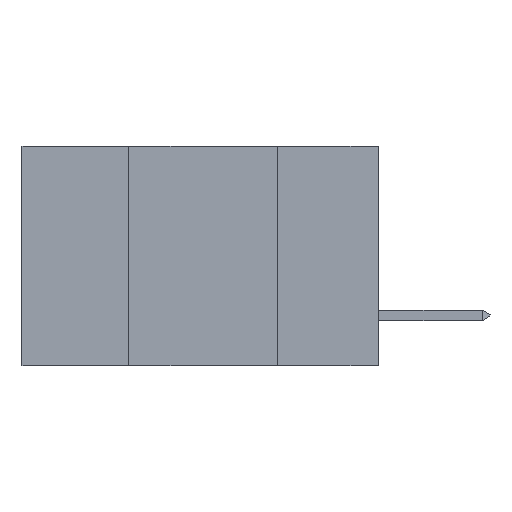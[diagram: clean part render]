
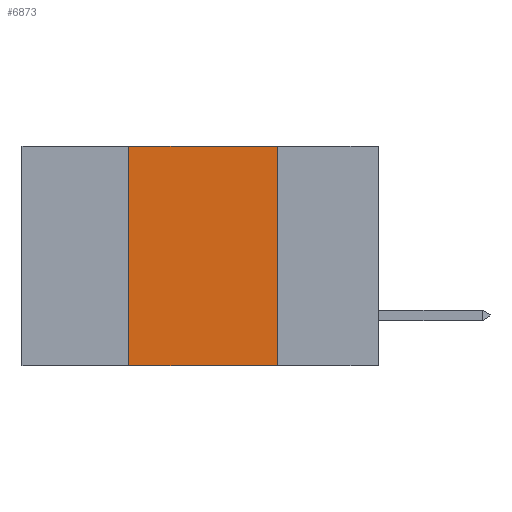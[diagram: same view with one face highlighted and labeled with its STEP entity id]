
A CAD part, left-side view. The second image highlights one B-rep face of the part: STEP entity #6873.
In plain terms, the highlighted planar face has unit normal (-1, 0, 0).
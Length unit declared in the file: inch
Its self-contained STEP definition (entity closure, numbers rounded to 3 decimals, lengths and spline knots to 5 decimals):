
#1115 = DIRECTION ( 'NONE',  ( 0., -1., 0. ) ) ;
#1425 = VECTOR ( 'NONE', #1115, 39.37008 ) ;
#1634 = ORIENTED_EDGE ( 'NONE', *, *, #8577, .F. ) ;
#1791 = DIRECTION ( 'NONE',  ( 1., 0., 0. ) ) ;
#1984 = LINE ( 'NONE', #8773, #12831 ) ;
#2904 = EDGE_LOOP ( 'NONE', ( #7566, #4981, #1634, #4426 ) ) ;
#3350 = LINE ( 'NONE', #6710, #7924 ) ;
#3454 = CARTESIAN_POINT ( 'NONE',  ( 0., 0.17, -0.37 ) ) ;
#4167 = VERTEX_POINT ( 'NONE', #10477 ) ;
#4426 = ORIENTED_EDGE ( 'NONE', *, *, #5807, .T. ) ;
#4702 = EDGE_CURVE ( 'NONE', #9043, #11125, #3350, .T. ) ;
#4981 = ORIENTED_EDGE ( 'NONE', *, *, #7376, .F. ) ;
#5735 = DIRECTION ( 'NONE',  ( 0., 0., 1. ) ) ;
#5807 = EDGE_CURVE ( 'NONE', #4167, #11125, #9439, .T. ) ;
#5879 = DIRECTION ( 'NONE',  ( 0., -1., 0. ) ) ;
#6710 = CARTESIAN_POINT ( 'NONE',  ( 0., 0.17, 0. ) ) ;
#6873 = ADVANCED_FACE ( 'NONE', ( #12068 ), #12814, .F. ) ;
#7376 = EDGE_CURVE ( 'NONE', #10424, #9043, #8310, .T. ) ;
#7560 = AXIS2_PLACEMENT_3D ( 'NONE', #8784, #1791, #7772 ) ;
#7566 = ORIENTED_EDGE ( 'NONE', *, *, #4702, .F. ) ;
#7772 = DIRECTION ( 'NONE',  ( 0., 0., -1. ) ) ;
#7924 = VECTOR ( 'NONE', #10723, 39.37008 ) ;
#8282 = CARTESIAN_POINT ( 'NONE',  ( 0., 0.17, 0. ) ) ;
#8310 = LINE ( 'NONE', #12990, #12689 ) ;
#8577 = EDGE_CURVE ( 'NONE', #4167, #10424, #1984, .T. ) ;
#8773 = CARTESIAN_POINT ( 'NONE',  ( 0., 0.42, 0. ) ) ;
#8784 = CARTESIAN_POINT ( 'NONE',  ( 0., 0.6, 0. ) ) ;
#9043 = VERTEX_POINT ( 'NONE', #8282 ) ;
#9439 = LINE ( 'NONE', #11119, #1425 ) ;
#9812 = CARTESIAN_POINT ( 'NONE',  ( 0., 0.42, 0. ) ) ;
#10424 = VERTEX_POINT ( 'NONE', #9812 ) ;
#10477 = CARTESIAN_POINT ( 'NONE',  ( 0., 0.42, -0.37 ) ) ;
#10723 = DIRECTION ( 'NONE',  ( 0., 0., -1. ) ) ;
#11119 = CARTESIAN_POINT ( 'NONE',  ( 0., 0.6, -0.37 ) ) ;
#11125 = VERTEX_POINT ( 'NONE', #3454 ) ;
#12068 = FACE_OUTER_BOUND ( 'NONE', #2904, .T. ) ;
#12689 = VECTOR ( 'NONE', #5879, 39.37008 ) ;
#12814 = PLANE ( 'NONE',  #7560 ) ;
#12831 = VECTOR ( 'NONE', #5735, 39.37008 ) ;
#12990 = CARTESIAN_POINT ( 'NONE',  ( 0., 0.6, 0. ) ) ;
